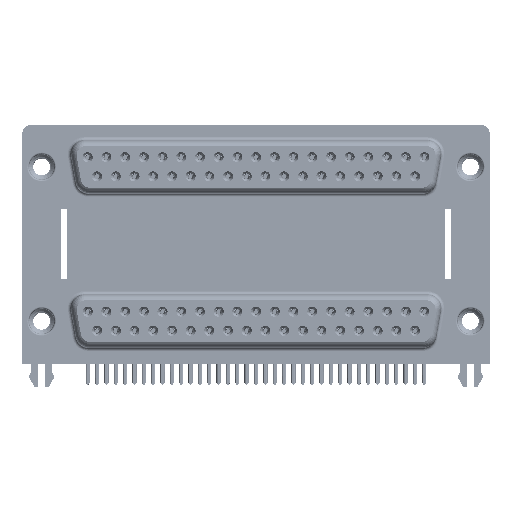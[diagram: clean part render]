
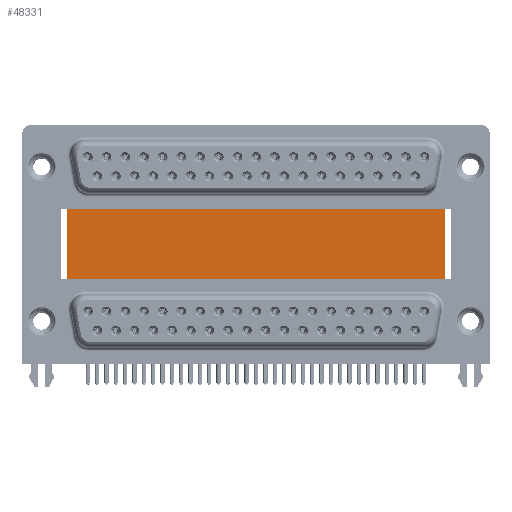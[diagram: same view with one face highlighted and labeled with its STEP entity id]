
A CAD part, top view. The second image highlights one B-rep face of the part: STEP entity #48331.
In plain terms, the highlighted planar face has unit normal (0, 0, 1).
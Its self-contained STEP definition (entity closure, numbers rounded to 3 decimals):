
#320 = ORIENTED_EDGE ( 'NONE', *, *, #56638, .F. ) ;
#1016 = CARTESIAN_POINT ( 'NONE',  ( 3.79, -3.735, -12. ) ) ;
#1756 = FACE_OUTER_BOUND ( 'NONE', #68239, .T. ) ;
#2000 = LINE ( 'NONE', #25570, #70036 ) ;
#3987 = DIRECTION ( 'NONE',  ( 1., 0., 0. ) ) ;
#4021 = VECTOR ( 'NONE', #65451, 1000. ) ;
#10728 = CARTESIAN_POINT ( 'NONE',  ( 59.71, -3.735, -12. ) ) ;
#13464 = ORIENTED_EDGE ( 'NONE', *, *, #21656, .F. ) ;
#15515 = VERTEX_POINT ( 'NONE', #53718 ) ;
#15577 = LINE ( 'NONE', #38774, #72066 ) ;
#17308 = VERTEX_POINT ( 'NONE', #34632 ) ;
#17519 = VERTEX_POINT ( 'NONE', #1016 ) ;
#19521 = DIRECTION ( 'NONE',  ( -1., 0., 0. ) ) ;
#19633 = LINE ( 'NONE', #43201, #45015 ) ;
#19772 = DIRECTION ( 'NONE',  ( 1., 0., 0. ) ) ;
#21369 = VERTEX_POINT ( 'NONE', #10728 ) ;
#21656 = EDGE_CURVE ( 'NONE', #17308, #15515, #15577, .T. ) ;
#25570 = CARTESIAN_POINT ( 'NONE',  ( 3.79, -3.735, -12. ) ) ;
#28655 = EDGE_CURVE ( 'NONE', #17308, #17519, #19633, .T. ) ;
#29275 = ORIENTED_EDGE ( 'NONE', *, *, #28655, .T. ) ;
#34632 = CARTESIAN_POINT ( 'NONE',  ( 3.79, 16.585, -12. ) ) ;
#38774 = CARTESIAN_POINT ( 'NONE',  ( 3.79, 16.585, -12. ) ) ;
#41160 = EDGE_CURVE ( 'NONE', #17519, #21369, #2000, .T. ) ;
#41912 = CARTESIAN_POINT ( 'NONE',  ( 59.71, 16.585, -12. ) ) ;
#43201 = CARTESIAN_POINT ( 'NONE',  ( 3.79, 16.585, -12. ) ) ;
#45015 = VECTOR ( 'NONE', #66737, 1000. ) ;
#48331 = ADVANCED_FACE ( 'NONE', ( #1756 ), #61617, .F. ) ;
#52361 = LINE ( 'NONE', #41912, #4021 ) ;
#53718 = CARTESIAN_POINT ( 'NONE',  ( 59.71, 16.585, -12. ) ) ;
#54576 = AXIS2_PLACEMENT_3D ( 'NONE', #73578, #67007, #19521 ) ;
#56638 = EDGE_CURVE ( 'NONE', #15515, #21369, #52361, .T. ) ;
#61617 = PLANE ( 'NONE',  #54576 ) ;
#65451 = DIRECTION ( 'NONE',  ( 0., -1., 0. ) ) ;
#66737 = DIRECTION ( 'NONE',  ( 0., -1., 0. ) ) ;
#67007 = DIRECTION ( 'NONE',  ( 0., 0., -1. ) ) ;
#68239 = EDGE_LOOP ( 'NONE', ( #75565, #320, #13464, #29275 ) ) ;
#70036 = VECTOR ( 'NONE', #19772, 1000. ) ;
#72066 = VECTOR ( 'NONE', #3987, 1000. ) ;
#73578 = CARTESIAN_POINT ( 'NONE',  ( 3.79, 16.585, -12. ) ) ;
#75565 = ORIENTED_EDGE ( 'NONE', *, *, #41160, .T. ) ;
